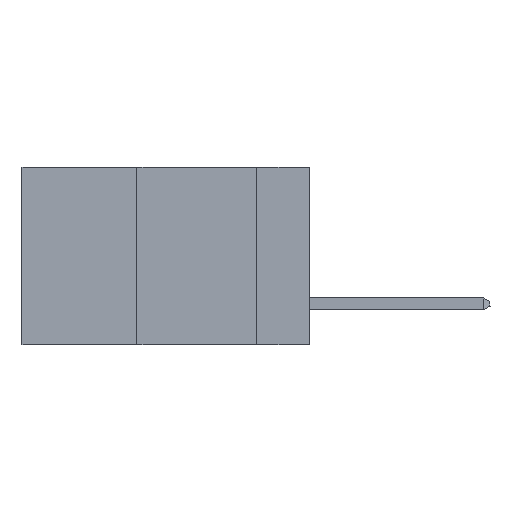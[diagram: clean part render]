
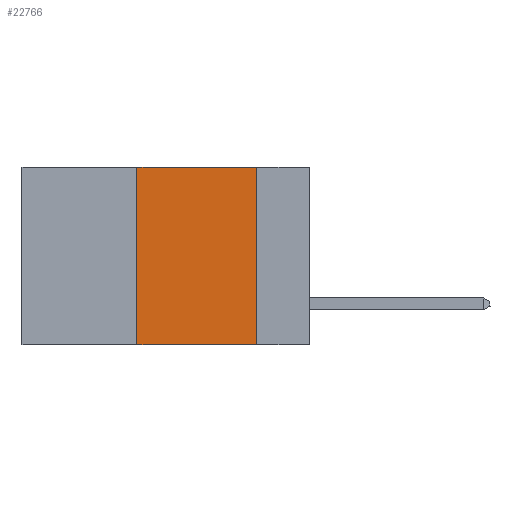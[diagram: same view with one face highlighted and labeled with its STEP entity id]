
A CAD part, left-side view. The second image highlights one B-rep face of the part: STEP entity #22766.
In plain terms, the highlighted planar face has unit normal (-1, 0, 0).
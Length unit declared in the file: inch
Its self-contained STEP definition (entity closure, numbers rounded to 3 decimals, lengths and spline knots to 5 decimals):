
#1543 = PLANE ( 'NONE',  #12259 ) ;
#2886 = LINE ( 'NONE', #6565, #23921 ) ;
#3102 = ORIENTED_EDGE ( 'NONE', *, *, #16514, .F. ) ;
#3272 = EDGE_CURVE ( 'NONE', #14364, #12992, #9420, .T. ) ;
#3381 = EDGE_CURVE ( 'NONE', #27696, #7385, #2886, .T. ) ;
#4496 = EDGE_LOOP ( 'NONE', ( #11539, #26733, #3102, #27217 ) ) ;
#5320 = CARTESIAN_POINT ( 'NONE',  ( 0., 0.11, 0. ) ) ;
#5598 = CARTESIAN_POINT ( 'NONE',  ( 0., 0.11, 0. ) ) ;
#6098 = VECTOR ( 'NONE', #16441, 39.37008 ) ;
#6565 = CARTESIAN_POINT ( 'NONE',  ( 0., 0.6, -0.37 ) ) ;
#7209 = EDGE_CURVE ( 'NONE', #12992, #7385, #17849, .T. ) ;
#7385 = VERTEX_POINT ( 'NONE', #11554 ) ;
#7815 = DIRECTION ( 'NONE',  ( 0., 0., 1. ) ) ;
#7919 = FACE_OUTER_BOUND ( 'NONE', #4496, .T. ) ;
#7938 = LINE ( 'NONE', #18929, #25189 ) ;
#9420 = LINE ( 'NONE', #20076, #19778 ) ;
#11539 = ORIENTED_EDGE ( 'NONE', *, *, #7209, .F. ) ;
#11554 = CARTESIAN_POINT ( 'NONE',  ( 0., 0.11, -0.37 ) ) ;
#12259 = AXIS2_PLACEMENT_3D ( 'NONE', #21585, #26032, #15124 ) ;
#12992 = VERTEX_POINT ( 'NONE', #5598 ) ;
#14364 = VERTEX_POINT ( 'NONE', #16825 ) ;
#15124 = DIRECTION ( 'NONE',  ( 0., 0., -1. ) ) ;
#16441 = DIRECTION ( 'NONE',  ( 0., 0., -1. ) ) ;
#16514 = EDGE_CURVE ( 'NONE', #27696, #14364, #7938, .T. ) ;
#16825 = CARTESIAN_POINT ( 'NONE',  ( 0., 0.36, 0. ) ) ;
#17849 = LINE ( 'NONE', #5320, #6098 ) ;
#18929 = CARTESIAN_POINT ( 'NONE',  ( 0., 0.36, 0. ) ) ;
#19778 = VECTOR ( 'NONE', #24306, 39.37008 ) ;
#20076 = CARTESIAN_POINT ( 'NONE',  ( 0., 0.6, 0. ) ) ;
#21585 = CARTESIAN_POINT ( 'NONE',  ( 0., 0.6, 0. ) ) ;
#22001 = DIRECTION ( 'NONE',  ( 0., -1., 0. ) ) ;
#22766 = ADVANCED_FACE ( 'NONE', ( #7919 ), #1543, .F. ) ;
#23921 = VECTOR ( 'NONE', #22001, 39.37008 ) ;
#24306 = DIRECTION ( 'NONE',  ( 0., -1., 0. ) ) ;
#24996 = CARTESIAN_POINT ( 'NONE',  ( 0., 0.36, -0.37 ) ) ;
#25189 = VECTOR ( 'NONE', #7815, 39.37008 ) ;
#26032 = DIRECTION ( 'NONE',  ( 1., 0., 0. ) ) ;
#26733 = ORIENTED_EDGE ( 'NONE', *, *, #3272, .F. ) ;
#27217 = ORIENTED_EDGE ( 'NONE', *, *, #3381, .T. ) ;
#27696 = VERTEX_POINT ( 'NONE', #24996 ) ;
